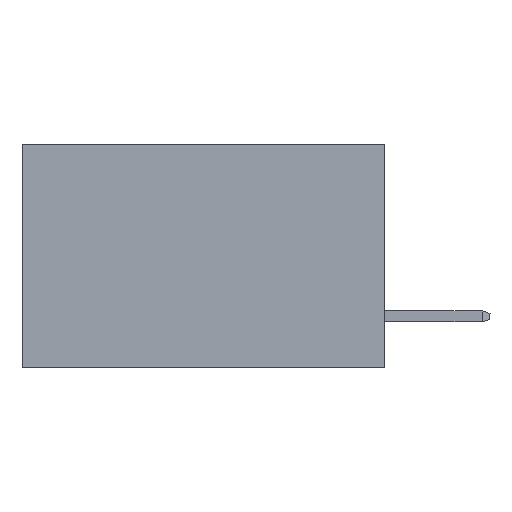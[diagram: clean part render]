
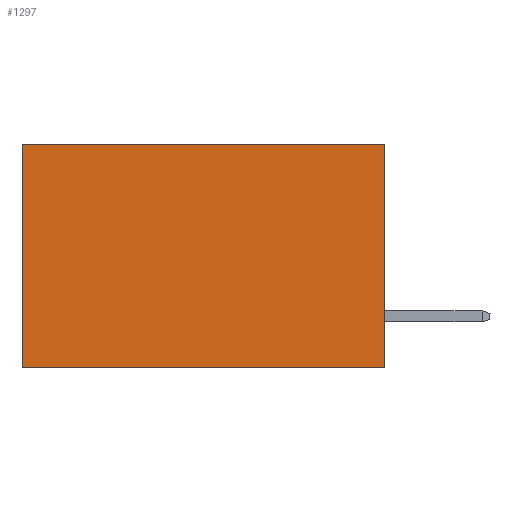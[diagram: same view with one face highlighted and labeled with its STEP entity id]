
A CAD part, left-side view. The second image highlights one B-rep face of the part: STEP entity #1297.
In plain terms, the highlighted planar face has unit normal (-1, 0, 0).
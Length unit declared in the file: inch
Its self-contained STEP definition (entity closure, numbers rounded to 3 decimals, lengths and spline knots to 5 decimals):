
#14 = CARTESIAN_POINT ( 'NONE',  ( 0.2615, 0., 0. ) ) ;
#367 = ORIENTED_EDGE ( 'NONE', *, *, #3870, .T. ) ;
#485 = EDGE_CURVE ( 'NONE', #3267, #2164, #3142, .T. ) ;
#734 = ORIENTED_EDGE ( 'NONE', *, *, #1104, .F. ) ;
#877 = VERTEX_POINT ( 'NONE', #6713 ) ;
#942 = EDGE_CURVE ( 'NONE', #877, #2164, #7292, .T. ) ;
#1104 = EDGE_CURVE ( 'NONE', #2257, #877, #1117, .T. ) ;
#1117 = LINE ( 'NONE', #7379, #2059 ) ;
#1163 = EDGE_LOOP ( 'NONE', ( #6176, #5841, #734, #367 ) ) ;
#1297 = ADVANCED_FACE ( 'NONE', ( #5304 ), #6657, .F. ) ;
#2059 = VECTOR ( 'NONE', #3056, 39.37008 ) ;
#2164 = VERTEX_POINT ( 'NONE', #2896 ) ;
#2184 = VECTOR ( 'NONE', #2607, 39.37008 ) ;
#2229 = CARTESIAN_POINT ( 'NONE',  ( 0.2615, 0., 0. ) ) ;
#2257 = VERTEX_POINT ( 'NONE', #14 ) ;
#2607 = DIRECTION ( 'NONE',  ( 0., 0., -1. ) ) ;
#2896 = CARTESIAN_POINT ( 'NONE',  ( 0.2615, 0.6, -0.37 ) ) ;
#3056 = DIRECTION ( 'NONE',  ( 0., 0., -1. ) ) ;
#3142 = LINE ( 'NONE', #4370, #2184 ) ;
#3267 = VERTEX_POINT ( 'NONE', #4539 ) ;
#3431 = CARTESIAN_POINT ( 'NONE',  ( 0.2615, 0., -0.37 ) ) ;
#3494 = DIRECTION ( 'NONE',  ( 0., 0., -1. ) ) ;
#3766 = VECTOR ( 'NONE', #5394, 39.37008 ) ;
#3870 = EDGE_CURVE ( 'NONE', #2257, #3267, #6745, .T. ) ;
#4124 = DIRECTION ( 'NONE',  ( 0., 1., 0. ) ) ;
#4370 = CARTESIAN_POINT ( 'NONE',  ( 0.2615, 0.6, -0.37 ) ) ;
#4539 = CARTESIAN_POINT ( 'NONE',  ( 0.2615, 0.6, 0. ) ) ;
#4681 = AXIS2_PLACEMENT_3D ( 'NONE', #6488, #6614, #3494 ) ;
#5304 = FACE_OUTER_BOUND ( 'NONE', #1163, .T. ) ;
#5394 = DIRECTION ( 'NONE',  ( 0., 1., 0. ) ) ;
#5722 = VECTOR ( 'NONE', #4124, 39.37008 ) ;
#5841 = ORIENTED_EDGE ( 'NONE', *, *, #942, .F. ) ;
#6176 = ORIENTED_EDGE ( 'NONE', *, *, #485, .T. ) ;
#6488 = CARTESIAN_POINT ( 'NONE',  ( 0.2615, 0., -0.37 ) ) ;
#6614 = DIRECTION ( 'NONE',  ( 1., 0., 0. ) ) ;
#6657 = PLANE ( 'NONE',  #4681 ) ;
#6713 = CARTESIAN_POINT ( 'NONE',  ( 0.2615, 0., -0.37 ) ) ;
#6745 = LINE ( 'NONE', #2229, #3766 ) ;
#7292 = LINE ( 'NONE', #3431, #5722 ) ;
#7379 = CARTESIAN_POINT ( 'NONE',  ( 0.2615, 0., -0.37 ) ) ;
